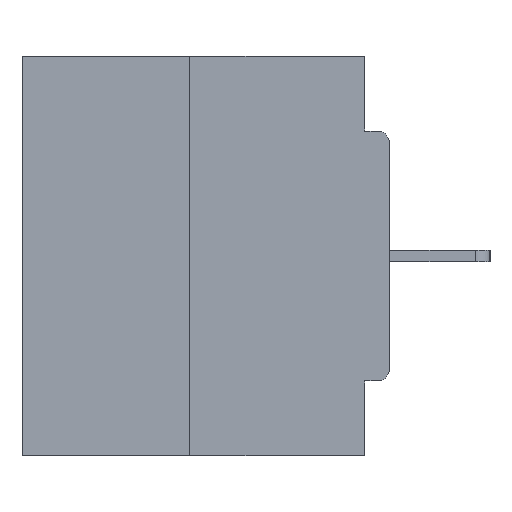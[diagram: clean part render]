
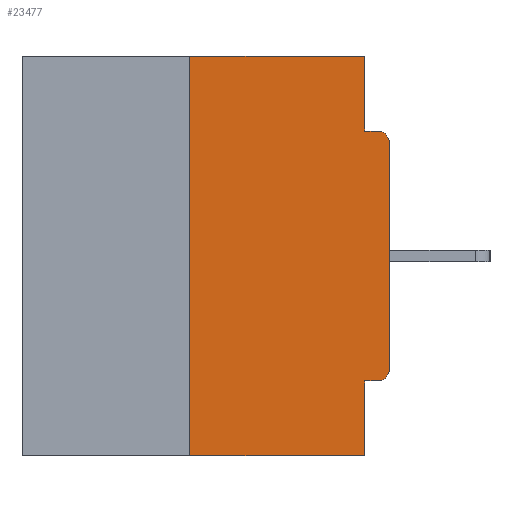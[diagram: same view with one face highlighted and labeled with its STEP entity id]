
A CAD part, left-side view. The second image highlights one B-rep face of the part: STEP entity #23477.
In plain terms, the highlighted planar face has unit normal (-1, 0, 0).
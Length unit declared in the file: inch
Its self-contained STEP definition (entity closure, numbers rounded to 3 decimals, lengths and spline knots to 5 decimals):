
#835 = VECTOR ( 'NONE', #7250, 39.37008 ) ;
#1081 = DIRECTION ( 'NONE',  ( 1., 0., 0. ) ) ;
#1403 = ORIENTED_EDGE ( 'NONE', *, *, #10982, .F. ) ;
#1430 = EDGE_CURVE ( 'NONE', #14305, #18432, #14353, .T. ) ;
#1716 = VERTEX_POINT ( 'NONE', #12093 ) ;
#1817 = EDGE_CURVE ( 'NONE', #27558, #14305, #11101, .T. ) ;
#2036 = DIRECTION ( 'NONE',  ( 0., -1., 0. ) ) ;
#2437 = CARTESIAN_POINT ( 'NONE',  ( 0., 0.25, 0. ) ) ;
#2927 = ORIENTED_EDGE ( 'NONE', *, *, #3283, .T. ) ;
#3283 = EDGE_CURVE ( 'NONE', #4840, #14360, #27061, .T. ) ;
#3880 = EDGE_CURVE ( 'NONE', #18432, #20606, #21371, .T. ) ;
#4578 = CARTESIAN_POINT ( 'NONE',  ( 0., 0., -0.4065 ) ) ;
#4840 = VERTEX_POINT ( 'NONE', #13478 ) ;
#4860 = VECTOR ( 'NONE', #23032, 39.37008 ) ;
#5404 = AXIS2_PLACEMENT_3D ( 'NONE', #13797, #29628, #16088 ) ;
#5652 = CARTESIAN_POINT ( 'NONE',  ( 0., 0.031, -0.0935 ) ) ;
#6409 = VERTEX_POINT ( 'NONE', #6497 ) ;
#6497 = CARTESIAN_POINT ( 'NONE',  ( 0., 0.25, -0.5 ) ) ;
#7235 = LINE ( 'NONE', #2437, #835 ) ;
#7250 = DIRECTION ( 'NONE',  ( 0., 0., 1. ) ) ;
#7942 = CARTESIAN_POINT ( 'NONE',  ( 0., 0., -0.0935 ) ) ;
#8048 = DIRECTION ( 'NONE',  ( -1., 0., 0. ) ) ;
#8502 = ORIENTED_EDGE ( 'NONE', *, *, #19425, .F. ) ;
#8677 = DIRECTION ( 'NONE',  ( 0., -1., 0. ) ) ;
#8764 = VECTOR ( 'NONE', #8677, 39.37008 ) ;
#9152 = VECTOR ( 'NONE', #28350, 39.37008 ) ;
#9512 = LINE ( 'NONE', #17783, #8764 ) ;
#9657 = VECTOR ( 'NONE', #2036, 39.37008 ) ;
#9806 = CARTESIAN_POINT ( 'NONE',  ( 0., 0., -0.1085 ) ) ;
#10982 = EDGE_CURVE ( 'NONE', #16396, #12559, #17189, .T. ) ;
#11101 = LINE ( 'NONE', #29187, #9657 ) ;
#11613 = CARTESIAN_POINT ( 'NONE',  ( 0., 0.031, -0.5 ) ) ;
#11825 = CARTESIAN_POINT ( 'NONE',  ( 0., 0.031, 0. ) ) ;
#12093 = CARTESIAN_POINT ( 'NONE',  ( 0., 0.015, -0.4065 ) ) ;
#12181 = CARTESIAN_POINT ( 'NONE',  ( 0., 0.031, -0.4065 ) ) ;
#12559 = VERTEX_POINT ( 'NONE', #29076 ) ;
#13478 = CARTESIAN_POINT ( 'NONE',  ( 0., 0., -0.3915 ) ) ;
#13797 = CARTESIAN_POINT ( 'NONE',  ( 0., 0.015, -0.3915 ) ) ;
#13889 = EDGE_CURVE ( 'NONE', #14360, #20606, #14553, .T. ) ;
#14068 = EDGE_CURVE ( 'NONE', #6409, #12559, #9512, .T. ) ;
#14305 = VERTEX_POINT ( 'NONE', #11825 ) ;
#14353 = LINE ( 'NONE', #18867, #25771 ) ;
#14360 = VERTEX_POINT ( 'NONE', #9806 ) ;
#14463 = AXIS2_PLACEMENT_3D ( 'NONE', #21832, #8048, #24127 ) ;
#14553 = CIRCLE ( 'NONE', #14463, 0.015 ) ;
#15168 = CARTESIAN_POINT ( 'NONE',  ( 0., 0.46, 0. ) ) ;
#15439 = CIRCLE ( 'NONE', #5404, 0.015 ) ;
#15575 = EDGE_CURVE ( 'NONE', #6409, #27558, #7235, .T. ) ;
#15997 = LINE ( 'NONE', #4578, #21380 ) ;
#16073 = ORIENTED_EDGE ( 'NONE', *, *, #13889, .T. ) ;
#16088 = DIRECTION ( 'NONE',  ( 0., 0., -1. ) ) ;
#16396 = VERTEX_POINT ( 'NONE', #12181 ) ;
#17189 = LINE ( 'NONE', #11613, #4860 ) ;
#17253 = AXIS2_PLACEMENT_3D ( 'NONE', #15168, #1081, #17422 ) ;
#17285 = DIRECTION ( 'NONE',  ( 0., 0., 1. ) ) ;
#17422 = DIRECTION ( 'NONE',  ( 0., 0., -1. ) ) ;
#17783 = CARTESIAN_POINT ( 'NONE',  ( 0., 0.46, -0.5 ) ) ;
#18432 = VERTEX_POINT ( 'NONE', #5652 ) ;
#18867 = CARTESIAN_POINT ( 'NONE',  ( 0., 0.031, 0. ) ) ;
#19091 = EDGE_LOOP ( 'NONE', ( #22526, #29839, #19269, #1403, #8502, #20736, #2927, #16073, #22167, #29520 ) ) ;
#19269 = ORIENTED_EDGE ( 'NONE', *, *, #14068, .T. ) ;
#19425 = EDGE_CURVE ( 'NONE', #1716, #16396, #15997, .T. ) ;
#19588 = VECTOR ( 'NONE', #17285, 39.37008 ) ;
#20606 = VERTEX_POINT ( 'NONE', #25606 ) ;
#20736 = ORIENTED_EDGE ( 'NONE', *, *, #23120, .T. ) ;
#21371 = LINE ( 'NONE', #7942, #9152 ) ;
#21380 = VECTOR ( 'NONE', #25475, 39.37008 ) ;
#21832 = CARTESIAN_POINT ( 'NONE',  ( 0., 0.015, -0.1085 ) ) ;
#22167 = ORIENTED_EDGE ( 'NONE', *, *, #3880, .F. ) ;
#22526 = ORIENTED_EDGE ( 'NONE', *, *, #1817, .F. ) ;
#22649 = DIRECTION ( 'NONE',  ( 0., 0., -1. ) ) ;
#23032 = DIRECTION ( 'NONE',  ( 0., 0., -1. ) ) ;
#23120 = EDGE_CURVE ( 'NONE', #1716, #4840, #15439, .T. ) ;
#23477 = ADVANCED_FACE ( 'NONE', ( #28886 ), #28751, .F. ) ;
#24127 = DIRECTION ( 'NONE',  ( 0., 0., -1. ) ) ;
#25247 = CARTESIAN_POINT ( 'NONE',  ( 0., 0.25, 0. ) ) ;
#25475 = DIRECTION ( 'NONE',  ( 0., 1., 0. ) ) ;
#25606 = CARTESIAN_POINT ( 'NONE',  ( 0., 0.015, -0.0935 ) ) ;
#25771 = VECTOR ( 'NONE', #22649, 39.37008 ) ;
#27061 = LINE ( 'NONE', #27630, #19588 ) ;
#27558 = VERTEX_POINT ( 'NONE', #25247 ) ;
#27630 = CARTESIAN_POINT ( 'NONE',  ( 0., 0., 0. ) ) ;
#28350 = DIRECTION ( 'NONE',  ( 0., -1., 0. ) ) ;
#28751 = PLANE ( 'NONE',  #17253 ) ;
#28886 = FACE_OUTER_BOUND ( 'NONE', #19091, .T. ) ;
#29076 = CARTESIAN_POINT ( 'NONE',  ( 0., 0.031, -0.5 ) ) ;
#29187 = CARTESIAN_POINT ( 'NONE',  ( 0., 0.46, 0. ) ) ;
#29520 = ORIENTED_EDGE ( 'NONE', *, *, #1430, .F. ) ;
#29628 = DIRECTION ( 'NONE',  ( -1., 0., 0. ) ) ;
#29839 = ORIENTED_EDGE ( 'NONE', *, *, #15575, .F. ) ;
